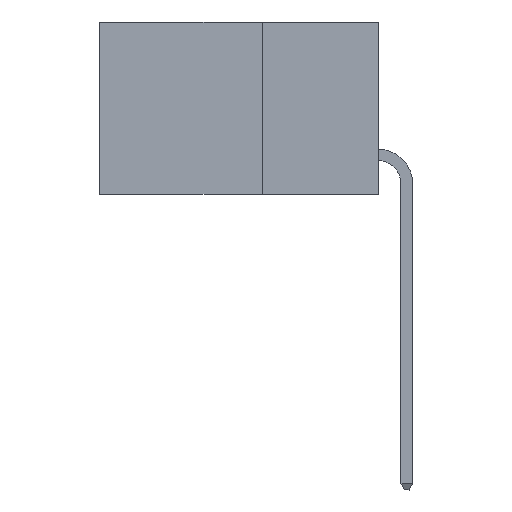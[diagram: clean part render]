
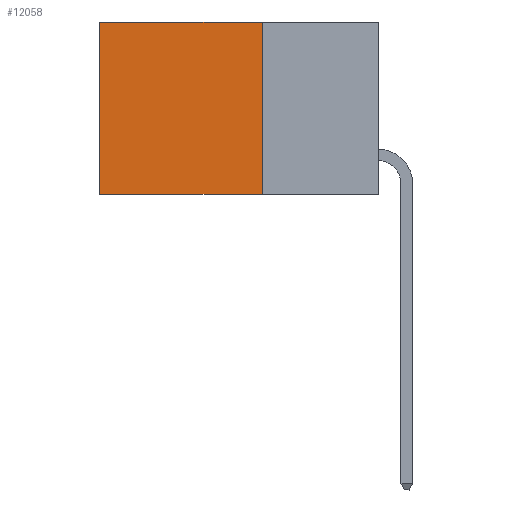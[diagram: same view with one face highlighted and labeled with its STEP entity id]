
A CAD part, left-side view. The second image highlights one B-rep face of the part: STEP entity #12058.
In plain terms, the highlighted planar face has unit normal (-1, 0, 0).
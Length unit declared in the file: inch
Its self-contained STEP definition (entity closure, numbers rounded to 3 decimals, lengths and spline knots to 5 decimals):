
#208 = EDGE_CURVE ( 'NONE', #3988, #3388, #8708, .T. ) ;
#721 = VERTEX_POINT ( 'NONE', #1443 ) ;
#1329 = AXIS2_PLACEMENT_3D ( 'NONE', #14443, #7094, #9485 ) ;
#1443 = CARTESIAN_POINT ( 'NONE',  ( 0.2615, 0.25, 0. ) ) ;
#1565 = CARTESIAN_POINT ( 'NONE',  ( 0.2615, 0.25, 0. ) ) ;
#2258 = LINE ( 'NONE', #3238, #10227 ) ;
#2277 = DIRECTION ( 'NONE',  ( 0., 1., 0. ) ) ;
#3238 = CARTESIAN_POINT ( 'NONE',  ( 0.2615, 0.25, -0.37 ) ) ;
#3388 = VERTEX_POINT ( 'NONE', #4539 ) ;
#3988 = VERTEX_POINT ( 'NONE', #13762 ) ;
#4408 = CARTESIAN_POINT ( 'NONE',  ( 0.2615, 0.6, -0.37 ) ) ;
#4445 = ORIENTED_EDGE ( 'NONE', *, *, #208, .F. ) ;
#4539 = CARTESIAN_POINT ( 'NONE',  ( 0.2615, 0.6, -0.37 ) ) ;
#4708 = EDGE_CURVE ( 'NONE', #721, #4980, #12806, .T. ) ;
#4862 = EDGE_CURVE ( 'NONE', #4980, #3388, #14406, .T. ) ;
#4980 = VERTEX_POINT ( 'NONE', #13429 ) ;
#5327 = DIRECTION ( 'NONE',  ( 0., 1., 0. ) ) ;
#5693 = PLANE ( 'NONE',  #1329 ) ;
#6451 = ORIENTED_EDGE ( 'NONE', *, *, #4708, .T. ) ;
#6660 = VECTOR ( 'NONE', #2277, 39.37008 ) ;
#7094 = DIRECTION ( 'NONE',  ( 1., 0., 0. ) ) ;
#8185 = DIRECTION ( 'NONE',  ( 0., 0., -1. ) ) ;
#8668 = VECTOR ( 'NONE', #11752, 39.37008 ) ;
#8708 = LINE ( 'NONE', #13428, #6660 ) ;
#9485 = DIRECTION ( 'NONE',  ( 0., 0., -1. ) ) ;
#10227 = VECTOR ( 'NONE', #8185, 39.37008 ) ;
#10405 = EDGE_LOOP ( 'NONE', ( #14716, #4445, #14811, #6451 ) ) ;
#10484 = VECTOR ( 'NONE', #5327, 39.37008 ) ;
#10638 = FACE_OUTER_BOUND ( 'NONE', #10405, .T. ) ;
#11678 = EDGE_CURVE ( 'NONE', #721, #3988, #2258, .T. ) ;
#11752 = DIRECTION ( 'NONE',  ( 0., 0., -1. ) ) ;
#12058 = ADVANCED_FACE ( 'NONE', ( #10638 ), #5693, .F. ) ;
#12806 = LINE ( 'NONE', #1565, #10484 ) ;
#13428 = CARTESIAN_POINT ( 'NONE',  ( 0.2615, 0.25, -0.37 ) ) ;
#13429 = CARTESIAN_POINT ( 'NONE',  ( 0.2615, 0.6, 0. ) ) ;
#13762 = CARTESIAN_POINT ( 'NONE',  ( 0.2615, 0.25, -0.37 ) ) ;
#14406 = LINE ( 'NONE', #4408, #8668 ) ;
#14443 = CARTESIAN_POINT ( 'NONE',  ( 0.2615, 0.25, -0.37 ) ) ;
#14716 = ORIENTED_EDGE ( 'NONE', *, *, #4862, .T. ) ;
#14811 = ORIENTED_EDGE ( 'NONE', *, *, #11678, .F. ) ;
